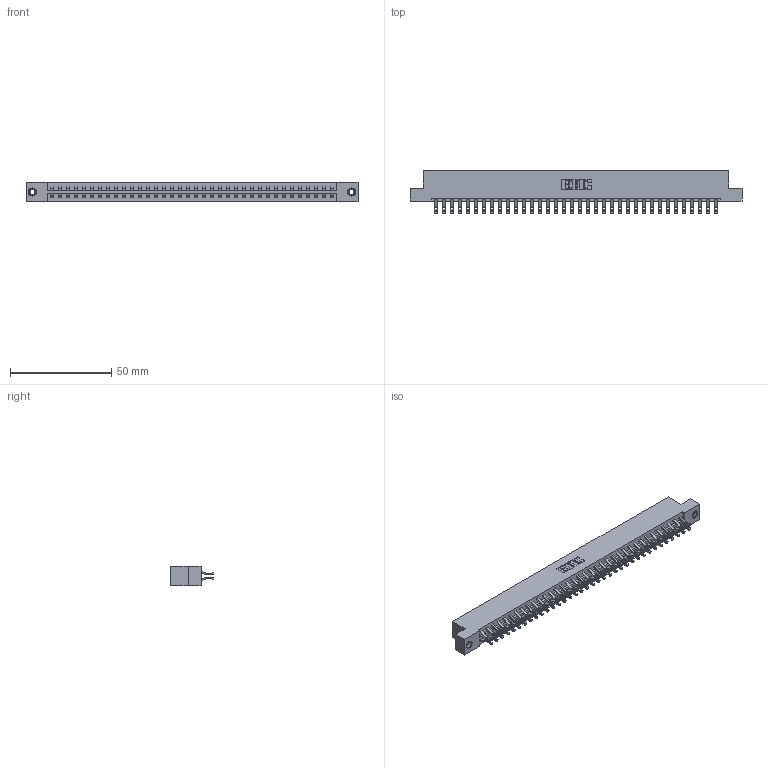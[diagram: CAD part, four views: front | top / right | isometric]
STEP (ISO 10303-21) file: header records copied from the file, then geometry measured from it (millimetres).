
FILE_DESCRIPTION (( 'STEP AP203' ), '1' );
FILE_NAME ('833-072-555-207.STEP', '2020-06-05T14:43:41', ( '' ), ( '' ), 'SwSTEP 2.0', 'SolidWorks 2020', '' );
FILE_SCHEMA (( 'CONFIG_CONTROL_DESIGN' ));
Length unit declared in the file: inch
Products named in the file (4): 833 Part_Flush - .156 Dia - TI; 833-072-555-207; 345-250-001_345-250-005-103; 345-292-001_555 Tail
Assembly tree (75 placements, depth 2):
  833-072-555-207
    833 Part_Flush - .156 Dia - TI
    345-292-001_555 Tail  x72
    345-250-001_345-250-005-103  x2
Bounding box: 164.19 x 21.47 x 9.4 mm (x, y, z)
Volume: 16901.6 mm3; surface area: 20732.6 mm2
Topology: 75 solids, 75 shells, 4350 faces, 13623 edges, 9074 vertices
Faces by surface type: plane 2550, cylinder 1784, cone 12, torus 4
Entity records: 25448 total; most frequent: CARTESIAN_POINT 4243, ORIENTED_EDGE 4142, DIRECTION 3637, EDGE_CURVE 2071, LINE 1903, VECTOR 1903, VERTEX_POINT 1376, AXIS2_PLACEMENT_3D 867
